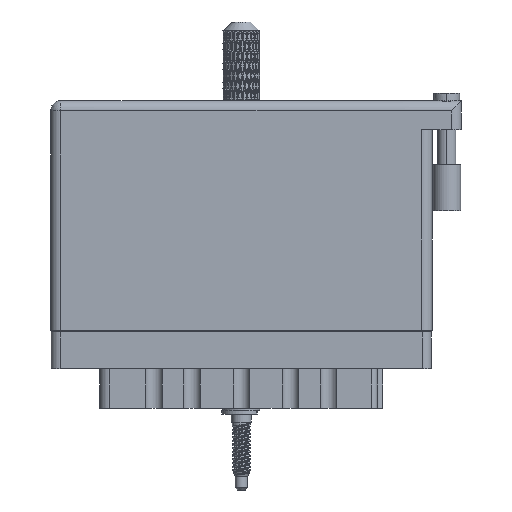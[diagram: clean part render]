
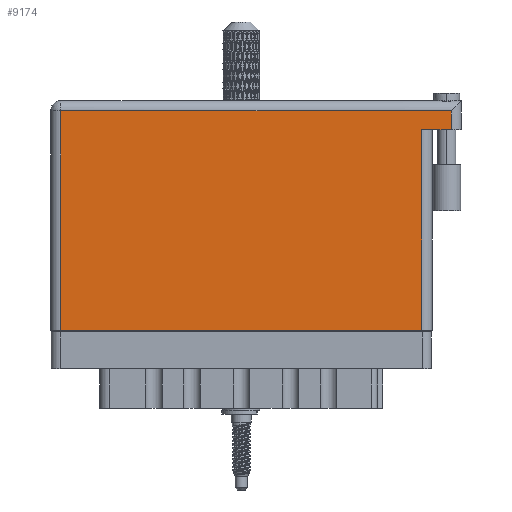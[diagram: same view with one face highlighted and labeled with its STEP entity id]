
A CAD part, front view. The second image highlights one B-rep face of the part: STEP entity #9174.
In plain terms, the highlighted face is planar.
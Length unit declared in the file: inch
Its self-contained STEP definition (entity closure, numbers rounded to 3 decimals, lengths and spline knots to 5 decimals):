
#6762 = CARTESIAN_POINT ( 'NONE',  ( 2.53, 1.369, 0. ) ) ;
#7026 = EDGE_CURVE ( 'NONE', #63385, #96797, #19563, .T. ) ;
#7712 = DIRECTION ( 'NONE',  ( -1., 0., 0. ) ) ;
#7895 = EDGE_CURVE ( 'NONE', #61518, #30670, #109844, .T. ) ;
#8444 = EDGE_CURVE ( 'NONE', #61167, #63385, #95345, .T. ) ;
#9174 = ADVANCED_FACE ( 'NONE', ( #88107 ), #32449, .F. ) ;
#9920 = LINE ( 'NONE', #109816, #106301 ) ;
#10701 = ORIENTED_EDGE ( 'NONE', *, *, #7026, .T. ) ;
#15165 = DIRECTION ( 'NONE',  ( 0., 0., -1. ) ) ;
#16820 = ORIENTED_EDGE ( 'NONE', *, *, #36222, .F. ) ;
#19563 = LINE ( 'NONE', #6762, #45299 ) ;
#19783 = LINE ( 'NONE', #77982, #50052 ) ;
#24777 = CARTESIAN_POINT ( 'NONE',  ( 2.73, 1.566, 0. ) ) ;
#25291 = DIRECTION ( 'NONE',  ( 0., 1., 0. ) ) ;
#25620 = VECTOR ( 'NONE', #87792, 39.37008 ) ;
#28817 = EDGE_LOOP ( 'NONE', ( #99934, #10701, #16820, #52011, #30772, #78692 ) ) ;
#29150 = DIRECTION ( 'NONE',  ( 0., -1., 0. ) ) ;
#30670 = VERTEX_POINT ( 'NONE', #78689 ) ;
#30772 = ORIENTED_EDGE ( 'NONE', *, *, #7895, .T. ) ;
#32449 = PLANE ( 'NONE',  #84267 ) ;
#32823 = CARTESIAN_POINT ( 'NONE',  ( 0., 1.566, 0. ) ) ;
#35820 = EDGE_CURVE ( 'NONE', #83043, #61518, #117468, .T. ) ;
#36222 = EDGE_CURVE ( 'NONE', #83043, #96797, #19783, .T. ) ;
#43225 = CARTESIAN_POINT ( 'NONE',  ( 2.53, 0., 0. ) ) ;
#45299 = VECTOR ( 'NONE', #25291, 39.37008 ) ;
#50052 = VECTOR ( 'NONE', #69580, 39.37008 ) ;
#52011 = ORIENTED_EDGE ( 'NONE', *, *, #35820, .T. ) ;
#53778 = CARTESIAN_POINT ( 'NONE',  ( 0.07, 0., 0. ) ) ;
#61167 = VERTEX_POINT ( 'NONE', #53778 ) ;
#61518 = VERTEX_POINT ( 'NONE', #81009 ) ;
#62716 = CARTESIAN_POINT ( 'NONE',  ( 0., 1.496, 0. ) ) ;
#62775 = CARTESIAN_POINT ( 'NONE',  ( 2.53, 1.369, 0. ) ) ;
#63385 = VERTEX_POINT ( 'NONE', #43225 ) ;
#65247 = EDGE_CURVE ( 'NONE', #30670, #61167, #9920, .T. ) ;
#69580 = DIRECTION ( 'NONE',  ( -1., 0., 0. ) ) ;
#77982 = CARTESIAN_POINT ( 'NONE',  ( 2.8, 1.369, 0. ) ) ;
#78689 = CARTESIAN_POINT ( 'NONE',  ( 0.07, 1.496, 0. ) ) ;
#78692 = ORIENTED_EDGE ( 'NONE', *, *, #65247, .T. ) ;
#79315 = DIRECTION ( 'NONE',  ( -1., 0., 0. ) ) ;
#81009 = CARTESIAN_POINT ( 'NONE',  ( 2.73, 1.496, 0. ) ) ;
#83043 = VERTEX_POINT ( 'NONE', #103416 ) ;
#84267 = AXIS2_PLACEMENT_3D ( 'NONE', #32823, #15165, #79315 ) ;
#85319 = VECTOR ( 'NONE', #86581, 39.37008 ) ;
#85442 = VECTOR ( 'NONE', #7712, 39.37008 ) ;
#85787 = CARTESIAN_POINT ( 'NONE',  ( 0., 0., 0. ) ) ;
#86581 = DIRECTION ( 'NONE',  ( 1., 0., 0. ) ) ;
#87792 = DIRECTION ( 'NONE',  ( 0., 1., 0. ) ) ;
#88107 = FACE_OUTER_BOUND ( 'NONE', #28817, .T. ) ;
#95345 = LINE ( 'NONE', #85787, #85319 ) ;
#96797 = VERTEX_POINT ( 'NONE', #62775 ) ;
#99934 = ORIENTED_EDGE ( 'NONE', *, *, #8444, .T. ) ;
#103416 = CARTESIAN_POINT ( 'NONE',  ( 2.73, 1.369, 0. ) ) ;
#106301 = VECTOR ( 'NONE', #29150, 39.37008 ) ;
#109816 = CARTESIAN_POINT ( 'NONE',  ( 0.07, 0., 0. ) ) ;
#109844 = LINE ( 'NONE', #62716, #85442 ) ;
#117468 = LINE ( 'NONE', #24777, #25620 ) ;
